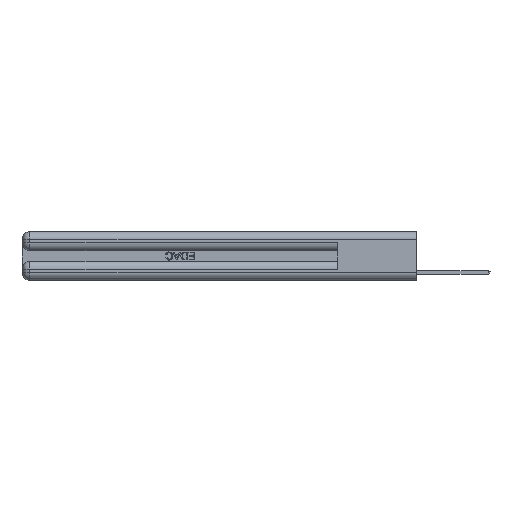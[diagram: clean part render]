
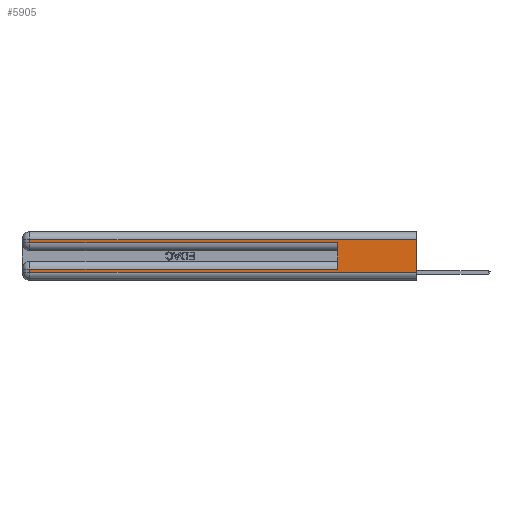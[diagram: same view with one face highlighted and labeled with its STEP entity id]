
A CAD part, left-side view. The second image highlights one B-rep face of the part: STEP entity #5905.
In plain terms, the highlighted planar face has unit normal (-1, 0, 0).
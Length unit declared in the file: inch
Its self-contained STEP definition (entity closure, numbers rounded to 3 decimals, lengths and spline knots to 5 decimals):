
#544 = CARTESIAN_POINT ( 'NONE',  ( 0., 2.94, 0.37 ) ) ;
#1764 = EDGE_CURVE ( 'NONE', #25260, #30531, #26524, .T. ) ;
#2196 = DIRECTION ( 'NONE',  ( 0., 0., -1. ) ) ;
#2561 = VECTOR ( 'NONE', #2196, 39.37008 ) ;
#3429 = CARTESIAN_POINT ( 'NONE',  ( 0., 2.94, 0.31 ) ) ;
#4288 = DIRECTION ( 'NONE',  ( 1., 0., 0. ) ) ;
#4749 = FACE_OUTER_BOUND ( 'NONE', #7462, .T. ) ;
#4850 = DIRECTION ( 'NONE',  ( 0., 1., 0. ) ) ;
#5133 = ORIENTED_EDGE ( 'NONE', *, *, #14481, .T. ) ;
#5400 = VECTOR ( 'NONE', #10881, 39.37008 ) ;
#5526 = ORIENTED_EDGE ( 'NONE', *, *, #14907, .T. ) ;
#5905 = ADVANCED_FACE ( 'NONE', ( #4749 ), #21654, .F. ) ;
#6430 = CARTESIAN_POINT ( 'NONE',  ( 0., 0.6, 0.285 ) ) ;
#6732 = VERTEX_POINT ( 'NONE', #3429 ) ;
#7297 = VECTOR ( 'NONE', #13746, 39.37008 ) ;
#7462 = EDGE_LOOP ( 'NONE', ( #27421, #20068, #5133, #5526, #29382, #26842, #14992, #25470 ) ) ;
#8677 = DIRECTION ( 'NONE',  ( 0., -1., 0. ) ) ;
#9441 = CARTESIAN_POINT ( 'NONE',  ( 0., 0., 0.37 ) ) ;
#9660 = DIRECTION ( 'NONE',  ( 0., 0., -1. ) ) ;
#9677 = CARTESIAN_POINT ( 'NONE',  ( 0., 2.94, 0.06 ) ) ;
#10171 = DIRECTION ( 'NONE',  ( 0., 0., -1. ) ) ;
#10881 = DIRECTION ( 'NONE',  ( 0., -1., 0. ) ) ;
#11690 = CARTESIAN_POINT ( 'NONE',  ( 0., 2.94, 0.085 ) ) ;
#11745 = AXIS2_PLACEMENT_3D ( 'NONE', #21021, #4288, #9660 ) ;
#12623 = VECTOR ( 'NONE', #14444, 39.37008 ) ;
#13211 = EDGE_CURVE ( 'NONE', #25260, #17766, #18338, .T. ) ;
#13722 = LINE ( 'NONE', #30788, #27803 ) ;
#13746 = DIRECTION ( 'NONE',  ( 0., 0., 1. ) ) ;
#14444 = DIRECTION ( 'NONE',  ( 0., 0., -1. ) ) ;
#14481 = EDGE_CURVE ( 'NONE', #6732, #28599, #22159, .T. ) ;
#14806 = CARTESIAN_POINT ( 'NONE',  ( 0., 0., 0.085 ) ) ;
#14874 = CARTESIAN_POINT ( 'NONE',  ( 0., 0.6, 0.085 ) ) ;
#14907 = EDGE_CURVE ( 'NONE', #28599, #17766, #18148, .T. ) ;
#14992 = ORIENTED_EDGE ( 'NONE', *, *, #19678, .T. ) ;
#15974 = VECTOR ( 'NONE', #10171, 39.37008 ) ;
#16266 = CARTESIAN_POINT ( 'NONE',  ( 0., 0.6, 0.145 ) ) ;
#17133 = VERTEX_POINT ( 'NONE', #9677 ) ;
#17752 = VERTEX_POINT ( 'NONE', #22891 ) ;
#17766 = VERTEX_POINT ( 'NONE', #6430 ) ;
#18148 = LINE ( 'NONE', #23360, #5400 ) ;
#18338 = LINE ( 'NONE', #16266, #7297 ) ;
#19197 = CARTESIAN_POINT ( 'NONE',  ( 0., 2.94, 0.37 ) ) ;
#19570 = VECTOR ( 'NONE', #24460, 39.37008 ) ;
#19678 = EDGE_CURVE ( 'NONE', #30531, #17133, #23952, .T. ) ;
#20068 = ORIENTED_EDGE ( 'NONE', *, *, #23854, .T. ) ;
#20438 = EDGE_CURVE ( 'NONE', #17133, #25033, #13722, .T. ) ;
#20511 = EDGE_CURVE ( 'NONE', #17752, #25033, #23839, .T. ) ;
#21021 = CARTESIAN_POINT ( 'NONE',  ( 0., 0., 0.37 ) ) ;
#21654 = PLANE ( 'NONE',  #11745 ) ;
#22159 = LINE ( 'NONE', #544, #15974 ) ;
#22891 = CARTESIAN_POINT ( 'NONE',  ( 0., 0., 0.31 ) ) ;
#22979 = CARTESIAN_POINT ( 'NONE',  ( 0., 0., 0.06 ) ) ;
#23360 = CARTESIAN_POINT ( 'NONE',  ( 0., 0., 0.285 ) ) ;
#23839 = LINE ( 'NONE', #9441, #2561 ) ;
#23854 = EDGE_CURVE ( 'NONE', #17752, #6732, #26522, .T. ) ;
#23952 = LINE ( 'NONE', #19197, #12623 ) ;
#24460 = DIRECTION ( 'NONE',  ( 0., 1., 0. ) ) ;
#24715 = CARTESIAN_POINT ( 'NONE',  ( 0., 2.94, 0.285 ) ) ;
#25033 = VERTEX_POINT ( 'NONE', #22979 ) ;
#25260 = VERTEX_POINT ( 'NONE', #14874 ) ;
#25470 = ORIENTED_EDGE ( 'NONE', *, *, #20438, .T. ) ;
#26522 = LINE ( 'NONE', #31097, #27455 ) ;
#26524 = LINE ( 'NONE', #14806, #19570 ) ;
#26842 = ORIENTED_EDGE ( 'NONE', *, *, #1764, .T. ) ;
#27421 = ORIENTED_EDGE ( 'NONE', *, *, #20511, .F. ) ;
#27455 = VECTOR ( 'NONE', #4850, 39.37008 ) ;
#27803 = VECTOR ( 'NONE', #8677, 39.37008 ) ;
#28599 = VERTEX_POINT ( 'NONE', #24715 ) ;
#29382 = ORIENTED_EDGE ( 'NONE', *, *, #13211, .F. ) ;
#30531 = VERTEX_POINT ( 'NONE', #11690 ) ;
#30788 = CARTESIAN_POINT ( 'NONE',  ( 0., 0., 0.06 ) ) ;
#31097 = CARTESIAN_POINT ( 'NONE',  ( 0., 0., 0.31 ) ) ;
